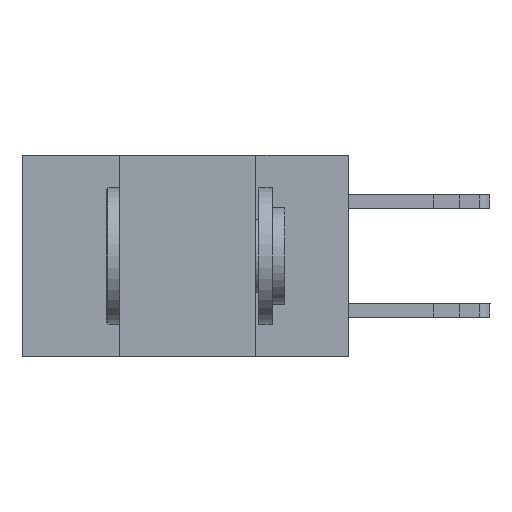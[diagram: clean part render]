
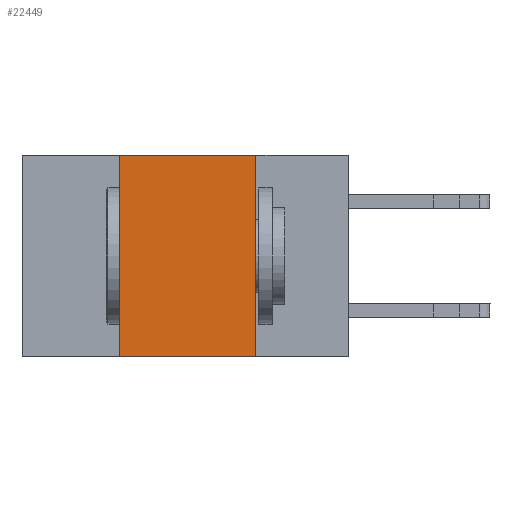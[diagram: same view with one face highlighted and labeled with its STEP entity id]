
A CAD part, left-side view. The second image highlights one B-rep face of the part: STEP entity #22449.
In plain terms, the highlighted planar face has unit normal (-1, 0, 0).
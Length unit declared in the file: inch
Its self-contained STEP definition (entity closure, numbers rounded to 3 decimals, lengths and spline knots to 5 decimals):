
#88 = DIRECTION ( 'NONE',  ( 0., -1., 0. ) ) ;
#1402 = DIRECTION ( 'NONE',  ( 0., 0., -1. ) ) ;
#1888 = EDGE_LOOP ( 'NONE', ( #3412, #21545, #15844, #16418 ) ) ;
#2080 = LINE ( 'NONE', #3594, #21781 ) ;
#2326 = DIRECTION ( 'NONE',  ( 0., 0., 1. ) ) ;
#3043 = DIRECTION ( 'NONE',  ( 0., -1., 0. ) ) ;
#3412 = ORIENTED_EDGE ( 'NONE', *, *, #15346, .F. ) ;
#3594 = CARTESIAN_POINT ( 'NONE',  ( 0., 0.6, -0.37 ) ) ;
#5414 = LINE ( 'NONE', #6468, #15138 ) ;
#6468 = CARTESIAN_POINT ( 'NONE',  ( 0., 0.17, 0. ) ) ;
#6937 = VERTEX_POINT ( 'NONE', #23351 ) ;
#7707 = CARTESIAN_POINT ( 'NONE',  ( 0., 0.42, 0. ) ) ;
#8007 = DIRECTION ( 'NONE',  ( 0., 0., -1. ) ) ;
#8587 = CARTESIAN_POINT ( 'NONE',  ( 0., 0.6, 0. ) ) ;
#10429 = DIRECTION ( 'NONE',  ( 1., 0., 0. ) ) ;
#11440 = EDGE_CURVE ( 'NONE', #6937, #21384, #16118, .T. ) ;
#11679 = CARTESIAN_POINT ( 'NONE',  ( 0., 0.6, 0. ) ) ;
#11775 = PLANE ( 'NONE',  #19703 ) ;
#12422 = EDGE_CURVE ( 'NONE', #21384, #15547, #22380, .T. ) ;
#12494 = CARTESIAN_POINT ( 'NONE',  ( 0., 0.17, 0. ) ) ;
#13142 = EDGE_CURVE ( 'NONE', #6937, #22150, #2080, .T. ) ;
#15138 = VECTOR ( 'NONE', #8007, 39.37008 ) ;
#15346 = EDGE_CURVE ( 'NONE', #15547, #22150, #5414, .T. ) ;
#15547 = VERTEX_POINT ( 'NONE', #12494 ) ;
#15844 = ORIENTED_EDGE ( 'NONE', *, *, #11440, .F. ) ;
#16118 = LINE ( 'NONE', #20533, #17260 ) ;
#16120 = VECTOR ( 'NONE', #3043, 39.37008 ) ;
#16418 = ORIENTED_EDGE ( 'NONE', *, *, #13142, .T. ) ;
#16766 = CARTESIAN_POINT ( 'NONE',  ( 0., 0.17, -0.37 ) ) ;
#17260 = VECTOR ( 'NONE', #2326, 39.37008 ) ;
#19703 = AXIS2_PLACEMENT_3D ( 'NONE', #8587, #10429, #1402 ) ;
#20261 = FACE_OUTER_BOUND ( 'NONE', #1888, .T. ) ;
#20533 = CARTESIAN_POINT ( 'NONE',  ( 0., 0.42, 0. ) ) ;
#21384 = VERTEX_POINT ( 'NONE', #7707 ) ;
#21545 = ORIENTED_EDGE ( 'NONE', *, *, #12422, .F. ) ;
#21781 = VECTOR ( 'NONE', #88, 39.37008 ) ;
#22150 = VERTEX_POINT ( 'NONE', #16766 ) ;
#22380 = LINE ( 'NONE', #11679, #16120 ) ;
#22449 = ADVANCED_FACE ( 'NONE', ( #20261 ), #11775, .F. ) ;
#23351 = CARTESIAN_POINT ( 'NONE',  ( 0., 0.42, -0.37 ) ) ;
